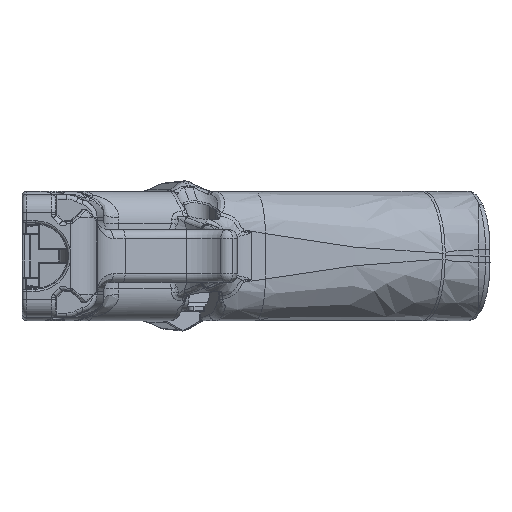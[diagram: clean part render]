
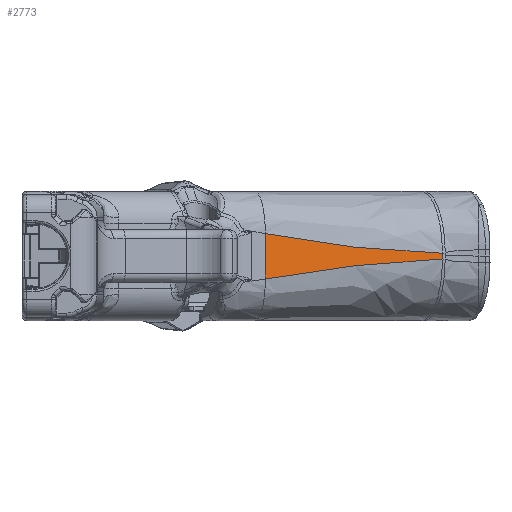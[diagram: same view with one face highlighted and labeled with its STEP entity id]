
A CAD part, left-side view. The second image highlights one B-rep face of the part: STEP entity #2773.
In plain terms, the highlighted cylindrical face has radius 450 mm (diameter 900 mm), a partial arc.
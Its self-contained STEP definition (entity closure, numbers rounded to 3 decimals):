
#981=CYLINDRICAL_SURFACE('',#23365,450.);
#2773=ADVANCED_FACE('',(#4439),#981,.T.);
#4439=FACE_OUTER_BOUND('',#5886,.T.);
#5886=EDGE_LOOP('',(#10360,#10361,#10362,#10363));
#7513=B_SPLINE_CURVE_WITH_KNOTS('',3,(#37881,#37882,#37883,#37884,#37885,
#37886,#37887,#37888,#37889,#37890,#37891,#37892,#37893,#37894,#37895,#37896,
#37897,#37898,#37899,#37900,#37901,#37902,#37903,#37904,#37905,#37906,#37907,
#37908,#37909,#37910,#37911,#37912,#37913,#37914,#37915,#37916,#37917,#37918),
 .UNSPECIFIED.,.F.,.F.,(4,2,2,1,2,2,1,1,2,2,2,2,1,1,2,2,2,2,1,2,2,4),(0.,
0.062,0.094,0.109,0.117,
0.125,0.187,0.219,0.234,
0.25,0.375,0.437,0.469,
0.484,0.492,0.5,0.625,
0.687,0.719,0.734,0.75,
1.),.UNSPECIFIED.);
#7514=B_SPLINE_CURVE_WITH_KNOTS('',3,(#37922,#37923,#37924,#37925,#37926,
#37927,#37928,#37929,#37930,#37931,#37932,#37933,#37934,#37935,#37936,#37937,
#37938,#37939,#37940,#37941,#37942,#37943,#37944,#37945,#37946,#37947,#37948,
#37949,#37950,#37951,#37952,#37953,#37954,#37955,#37956,#37957,#37958,#37959,
#37960,#37961,#37962,#37963,#37964),.UNSPECIFIED.,.F.,.F.,(4,2,2,2,1,2,
2,2,1,2,2,2,2,2,1,1,1,2,2,2,2,2,2,4),(0.,0.125,0.156,
0.187,0.25,0.312,0.375,
0.437,0.469,0.484,0.5,
0.625,0.75,0.812,0.844,
0.859,0.867,0.871,0.875,
0.906,0.922,0.93,0.937,
1.),.UNSPECIFIED.);
#10360=ORIENTED_EDGE('',*,*,#18414,.F.);
#10361=ORIENTED_EDGE('',*,*,#18415,.T.);
#10362=ORIENTED_EDGE('',*,*,#18416,.F.);
#10363=ORIENTED_EDGE('',*,*,#18417,.T.);
#16077=VERTEX_POINT('',#37879);
#16078=VERTEX_POINT('',#37880);
#16079=VERTEX_POINT('',#37919);
#16080=VERTEX_POINT('',#37921);
#18414=EDGE_CURVE('',#16077,#16078,#21051,.T.);
#18415=EDGE_CURVE('',#16077,#16079,#7513,.T.);
#18416=EDGE_CURVE('',#16080,#16079,#21052,.T.);
#18417=EDGE_CURVE('',#16080,#16078,#7514,.T.);
#21051=LINE('',#37878,#22117);
#21052=LINE('',#37920,#22118);
#22117=VECTOR('',#26729,1.);
#22118=VECTOR('',#26730,1.);
#23365=AXIS2_PLACEMENT_3D('',#37965,#26731,#26732);
#26729=DIRECTION('',(0.,0.,1.));
#26730=DIRECTION('',(0.,0.,-1.));
#26731=DIRECTION('',(0.,0.,1.));
#26732=DIRECTION('',(0.969,0.247,0.));
#37878=CARTESIAN_POINT('',(30.867,-11.345,-0.5));
#37879=CARTESIAN_POINT('',(30.867,-11.345,-5.696));
#37880=CARTESIAN_POINT('',(30.867,-11.345,4.594));
#37881=CARTESIAN_POINT('',(30.867,-11.345,-5.696));
#37882=CARTESIAN_POINT('',(31.033,-11.974,-5.609));
#37883=CARTESIAN_POINT('',(31.229,-12.716,-5.502));
#37884=CARTESIAN_POINT('',(31.573,-13.995,-5.313));
#37885=CARTESIAN_POINT('',(31.696,-14.45,-5.245));
#37886=CARTESIAN_POINT('',(31.893,-15.173,-5.136));
#37887=CARTESIAN_POINT('',(31.994,-15.545,-5.079));
#37888=CARTESIAN_POINT('',(32.101,-15.933,-5.02));
#37889=CARTESIAN_POINT('',(32.173,-16.194,-4.98));
#37890=CARTESIAN_POINT('',(32.217,-16.356,-4.955));
#37891=CARTESIAN_POINT('',(32.479,-17.304,-4.809));
#37892=CARTESIAN_POINT('',(32.831,-18.566,-4.614));
#37893=CARTESIAN_POINT('',(33.248,-20.036,-4.387));
#37894=CARTESIAN_POINT('',(33.428,-20.666,-4.29));
#37895=CARTESIAN_POINT('',(33.549,-21.086,-4.225));
#37896=CARTESIAN_POINT('',(33.598,-21.255,-4.198));
#37897=CARTESIAN_POINT('',(34.246,-23.503,-3.85));
#37898=CARTESIAN_POINT('',(34.791,-25.339,-3.573));
#37899=CARTESIAN_POINT('',(35.55,-27.851,-3.205));
#37900=CARTESIAN_POINT('',(35.794,-28.649,-3.091));
#37901=CARTESIAN_POINT('',(36.144,-29.785,-2.931));
#37902=CARTESIAN_POINT('',(36.316,-30.338,-2.854));
#37903=CARTESIAN_POINT('',(36.509,-30.957,-2.77));
#37904=CARTESIAN_POINT('',(36.59,-31.216,-2.735));
#37905=CARTESIAN_POINT('',(36.644,-31.388,-2.712));
#37906=CARTESIAN_POINT('',(36.661,-31.444,-2.704));
#37907=CARTESIAN_POINT('',(37.273,-33.39,-2.444));
#37908=CARTESIAN_POINT('',(37.834,-35.136,-2.23));
#37909=CARTESIAN_POINT('',(38.65,-37.628,-1.954));
#37910=CARTESIAN_POINT('',(38.917,-38.438,-1.869));
#37911=CARTESIAN_POINT('',(39.312,-39.62,-1.754));
#37912=CARTESIAN_POINT('',(39.507,-40.204,-1.699));
#37913=CARTESIAN_POINT('',(39.7,-40.775,-1.649));
#37914=CARTESIAN_POINT('',(39.828,-41.153,-1.616));
#37915=CARTESIAN_POINT('',(39.881,-41.307,-1.603));
#37916=CARTESIAN_POINT('',(41.154,-45.055,-1.294));
#37917=CARTESIAN_POINT('',(42.323,-48.355,-1.149));
#37918=CARTESIAN_POINT('',(43.449,-51.43,-1.15));
#37919=CARTESIAN_POINT('',(43.449,-51.43,-1.15));
#37920=CARTESIAN_POINT('',(43.449,-51.43,-0.5));
#37921=CARTESIAN_POINT('',(43.449,-51.43,0.15));
#37922=CARTESIAN_POINT('',(43.449,-51.43,0.15));
#37923=CARTESIAN_POINT('',(42.886,-49.893,0.148));
#37924=CARTESIAN_POINT('',(42.3,-48.264,0.18));
#37925=CARTESIAN_POINT('',(41.54,-46.111,0.26));
#37926=CARTESIAN_POINT('',(41.387,-45.675,0.278));
#37927=CARTESIAN_POINT('',(41.078,-44.791,0.319));
#37928=CARTESIAN_POINT('',(40.95,-44.423,0.337));
#37929=CARTESIAN_POINT('',(40.559,-43.295,0.399));
#37930=CARTESIAN_POINT('',(40.022,-41.732,0.498));
#37931=CARTESIAN_POINT('',(39.456,-40.052,0.631));
#37932=CARTESIAN_POINT('',(38.875,-38.311,0.781));
#37933=CARTESIAN_POINT('',(38.571,-37.391,0.866));
#37934=CARTESIAN_POINT('',(38.047,-35.786,1.026));
#37935=CARTESIAN_POINT('',(37.781,-34.965,1.112));
#37936=CARTESIAN_POINT('',(37.378,-33.708,1.253));
#37937=CARTESIAN_POINT('',(37.175,-33.072,1.326));
#37938=CARTESIAN_POINT('',(36.971,-32.427,1.403));
#37939=CARTESIAN_POINT('',(36.834,-31.994,1.455));
#37940=CARTESIAN_POINT('',(36.757,-31.748,1.485));
#37941=CARTESIAN_POINT('',(36.221,-30.04,1.696));
#37942=CARTESIAN_POINT('',(35.729,-28.445,1.908));
#37943=CARTESIAN_POINT('',(34.719,-25.097,2.382));
#37944=CARTESIAN_POINT('',(34.191,-23.311,2.648));
#37945=CARTESIAN_POINT('',(33.413,-20.616,3.069));
#37946=CARTESIAN_POINT('',(33.165,-19.745,3.207));
#37947=CARTESIAN_POINT('',(32.808,-18.48,3.41));
#37948=CARTESIAN_POINT('',(32.634,-17.858,3.511));
#37949=CARTESIAN_POINT('',(32.437,-17.15,3.627));
#37950=CARTESIAN_POINT('',(32.34,-16.801,3.685));
#37951=CARTESIAN_POINT('',(32.299,-16.652,3.71));
#37952=CARTESIAN_POINT('',(32.272,-16.553,3.726));
#37953=CARTESIAN_POINT('',(32.248,-16.468,3.74));
#37954=CARTESIAN_POINT('',(32.215,-16.349,3.76));
#37955=CARTESIAN_POINT('',(32.143,-16.088,3.804));
#37956=CARTESIAN_POINT('',(31.972,-15.462,3.91));
#37957=CARTESIAN_POINT('',(31.904,-15.214,3.951));
#37958=CARTESIAN_POINT('',(31.787,-14.785,4.024));
#37959=CARTESIAN_POINT('',(31.746,-14.631,4.05));
#37960=CARTESIAN_POINT('',(31.657,-14.306,4.105));
#37961=CARTESIAN_POINT('',(31.596,-14.079,4.143));
#37962=CARTESIAN_POINT('',(31.285,-12.926,4.337));
#37963=CARTESIAN_POINT('',(31.055,-12.057,4.481));
#37964=CARTESIAN_POINT('',(30.867,-11.345,4.594));
#37965=CARTESIAN_POINT('',(466.036,103.23,-0.5));
